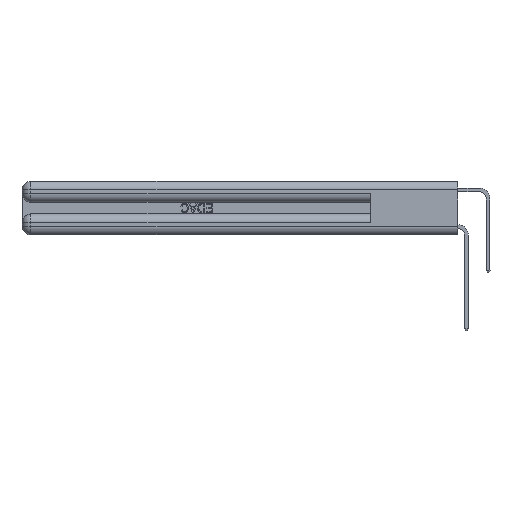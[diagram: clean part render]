
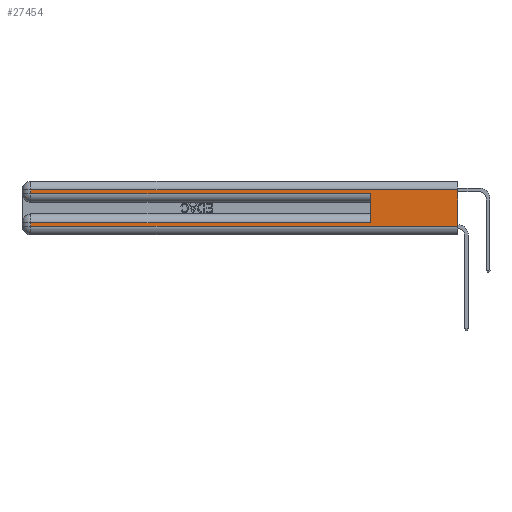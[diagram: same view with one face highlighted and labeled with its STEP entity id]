
A CAD part, left-side view. The second image highlights one B-rep face of the part: STEP entity #27454.
In plain terms, the highlighted planar face has unit normal (-1, 0, 0).
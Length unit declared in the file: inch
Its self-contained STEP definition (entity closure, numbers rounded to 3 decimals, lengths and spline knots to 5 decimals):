
#87 = CARTESIAN_POINT ( 'NONE',  ( 0., 0., 0.31 ) ) ;
#1055 = EDGE_LOOP ( 'NONE', ( #23758, #15916, #27271, #22618, #3590, #21228, #7885, #19299 ) ) ;
#2450 = CARTESIAN_POINT ( 'NONE',  ( 0., 0., 0.06 ) ) ;
#2523 = VERTEX_POINT ( 'NONE', #3877 ) ;
#2610 = CARTESIAN_POINT ( 'NONE',  ( 0., 2.94, 0.085 ) ) ;
#3084 = CARTESIAN_POINT ( 'NONE',  ( 0., 0., 0.085 ) ) ;
#3348 = CARTESIAN_POINT ( 'NONE',  ( 0., 0.6, 0.145 ) ) ;
#3548 = VECTOR ( 'NONE', #29403, 39.37008 ) ;
#3590 = ORIENTED_EDGE ( 'NONE', *, *, #18982, .F. ) ;
#3713 = CARTESIAN_POINT ( 'NONE',  ( 0., 0., 0.31 ) ) ;
#3877 = CARTESIAN_POINT ( 'NONE',  ( 0., 0.6, 0.285 ) ) ;
#4055 = EDGE_CURVE ( 'NONE', #18104, #2523, #28636, .T. ) ;
#4184 = VERTEX_POINT ( 'NONE', #2450 ) ;
#4392 = EDGE_CURVE ( 'NONE', #25534, #4184, #27341, .T. ) ;
#5663 = DIRECTION ( 'NONE',  ( 0., 1., 0. ) ) ;
#5744 = FACE_OUTER_BOUND ( 'NONE', #1055, .T. ) ;
#5992 = DIRECTION ( 'NONE',  ( 0., -1., 0. ) ) ;
#6061 = VECTOR ( 'NONE', #11065, 39.37008 ) ;
#7434 = VERTEX_POINT ( 'NONE', #2610 ) ;
#7546 = EDGE_CURVE ( 'NONE', #21968, #7434, #25716, .T. ) ;
#7817 = DIRECTION ( 'NONE',  ( 0., 0., -1. ) ) ;
#7885 = ORIENTED_EDGE ( 'NONE', *, *, #8793, .T. ) ;
#8486 = CARTESIAN_POINT ( 'NONE',  ( 0., 0., 0.37 ) ) ;
#8793 = EDGE_CURVE ( 'NONE', #7434, #23837, #19863, .T. ) ;
#9068 = DIRECTION ( 'NONE',  ( 0., -1., 0. ) ) ;
#9667 = VECTOR ( 'NONE', #5992, 39.37008 ) ;
#10187 = EDGE_CURVE ( 'NONE', #25534, #15195, #22116, .T. ) ;
#11065 = DIRECTION ( 'NONE',  ( 0., 0., 1. ) ) ;
#11904 = VECTOR ( 'NONE', #5663, 39.37008 ) ;
#12886 = VECTOR ( 'NONE', #7817, 39.37008 ) ;
#13034 = CARTESIAN_POINT ( 'NONE',  ( 0., 0., 0.37 ) ) ;
#13202 = DIRECTION ( 'NONE',  ( 0., 0., -1. ) ) ;
#15195 = VERTEX_POINT ( 'NONE', #27783 ) ;
#15916 = ORIENTED_EDGE ( 'NONE', *, *, #10187, .T. ) ;
#16107 = CARTESIAN_POINT ( 'NONE',  ( 0., 0., 0.06 ) ) ;
#18104 = VERTEX_POINT ( 'NONE', #21569 ) ;
#18211 = VECTOR ( 'NONE', #9068, 39.37008 ) ;
#18691 = CARTESIAN_POINT ( 'NONE',  ( 0., 0., 0.285 ) ) ;
#18982 = EDGE_CURVE ( 'NONE', #21968, #2523, #30316, .T. ) ;
#19104 = VECTOR ( 'NONE', #13202, 39.37008 ) ;
#19299 = ORIENTED_EDGE ( 'NONE', *, *, #28621, .T. ) ;
#19625 = LINE ( 'NONE', #28500, #3548 ) ;
#19709 = DIRECTION ( 'NONE',  ( 0., 1., 0. ) ) ;
#19863 = LINE ( 'NONE', #29642, #12886 ) ;
#21228 = ORIENTED_EDGE ( 'NONE', *, *, #7546, .T. ) ;
#21569 = CARTESIAN_POINT ( 'NONE',  ( 0., 2.94, 0.285 ) ) ;
#21968 = VERTEX_POINT ( 'NONE', #30910 ) ;
#22116 = LINE ( 'NONE', #87, #27807 ) ;
#22383 = CARTESIAN_POINT ( 'NONE',  ( 0., 2.94, 0.06 ) ) ;
#22618 = ORIENTED_EDGE ( 'NONE', *, *, #4055, .T. ) ;
#23409 = DIRECTION ( 'NONE',  ( 1., 0., 0. ) ) ;
#23758 = ORIENTED_EDGE ( 'NONE', *, *, #4392, .F. ) ;
#23837 = VERTEX_POINT ( 'NONE', #22383 ) ;
#25534 = VERTEX_POINT ( 'NONE', #3713 ) ;
#25716 = LINE ( 'NONE', #3084, #11904 ) ;
#25962 = DIRECTION ( 'NONE',  ( 0., 0., -1. ) ) ;
#26051 = LINE ( 'NONE', #16107, #9667 ) ;
#27271 = ORIENTED_EDGE ( 'NONE', *, *, #30135, .T. ) ;
#27341 = LINE ( 'NONE', #13034, #19104 ) ;
#27454 = ADVANCED_FACE ( 'NONE', ( #5744 ), #30764, .F. ) ;
#27783 = CARTESIAN_POINT ( 'NONE',  ( 0., 2.94, 0.31 ) ) ;
#27807 = VECTOR ( 'NONE', #19709, 39.37008 ) ;
#28500 = CARTESIAN_POINT ( 'NONE',  ( 0., 2.94, 0.37 ) ) ;
#28621 = EDGE_CURVE ( 'NONE', #23837, #4184, #26051, .T. ) ;
#28636 = LINE ( 'NONE', #18691, #18211 ) ;
#29071 = AXIS2_PLACEMENT_3D ( 'NONE', #8486, #23409, #25962 ) ;
#29403 = DIRECTION ( 'NONE',  ( 0., 0., -1. ) ) ;
#29642 = CARTESIAN_POINT ( 'NONE',  ( 0., 2.94, 0.37 ) ) ;
#30135 = EDGE_CURVE ( 'NONE', #15195, #18104, #19625, .T. ) ;
#30316 = LINE ( 'NONE', #3348, #6061 ) ;
#30764 = PLANE ( 'NONE',  #29071 ) ;
#30910 = CARTESIAN_POINT ( 'NONE',  ( 0., 0.6, 0.085 ) ) ;
